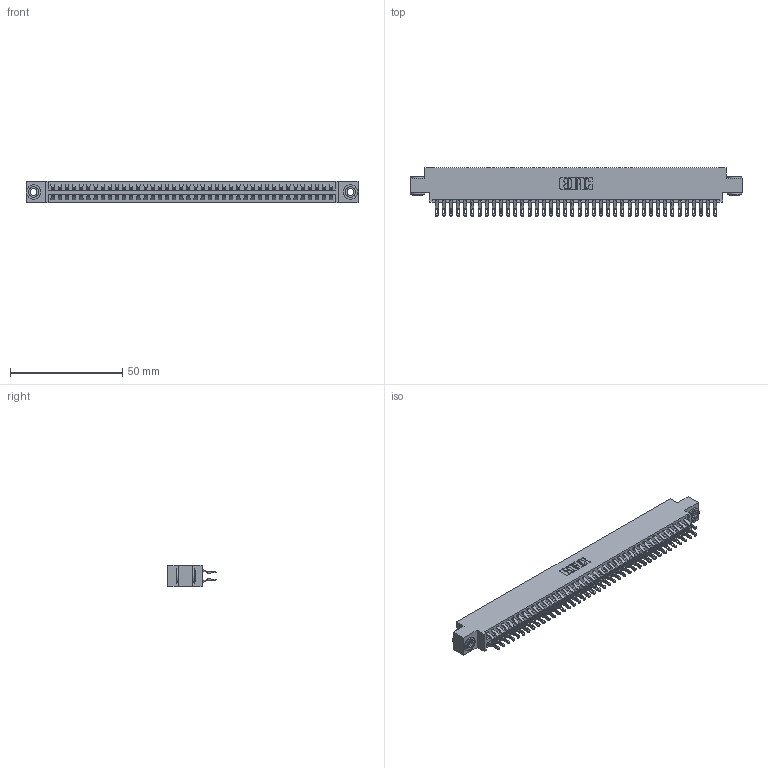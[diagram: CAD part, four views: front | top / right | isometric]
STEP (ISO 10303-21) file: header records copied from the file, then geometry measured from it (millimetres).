
FILE_DESCRIPTION (( 'STEP AP203' ), '1' );
FILE_NAME ('346-080-555-803.STEP', '2022-05-25T16:13:43', ( '' ), ( '' ), 'SwSTEP 2.0', 'SolidWorks 2020', '' );
FILE_SCHEMA (( 'CONFIG_CONTROL_DESIGN' ));
Length unit declared in the file: inch
Products named in the file (4): 345-250-002_345-250-002-102; 346 Part_0.170 Offset - 0.156 Dia-TH; 346-080-555-803; 345-292-001_555 Tail
Assembly tree (83 placements, depth 2):
  346-080-555-803
    346 Part_0.170 Offset - 0.156 Dia-TH
    345-292-001_555 Tail  x80
    345-250-002_345-250-002-102  x2
Bounding box: 147.57 x 21.46 x 9.4 mm (x, y, z)
Volume: 14453.5 mm3; surface area: 21091.4 mm2
Topology: 83 solids, 83 shells, 4818 faces, 15093 edges, 10058 vertices
Faces by surface type: plane 2744, cylinder 2066, cone 8
Entity records: 27898 total; most frequent: CARTESIAN_POINT 4619, ORIENTED_EDGE 4514, DIRECTION 4119, EDGE_CURVE 2257, VECTOR 1921, LINE 1921, VERTEX_POINT 1502, AXIS2_PLACEMENT_3D 1099
